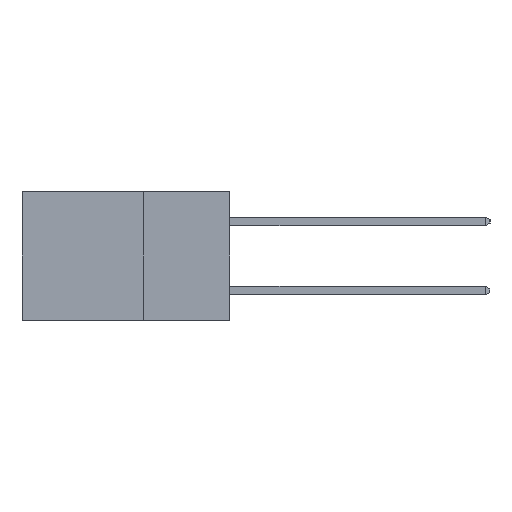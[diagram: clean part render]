
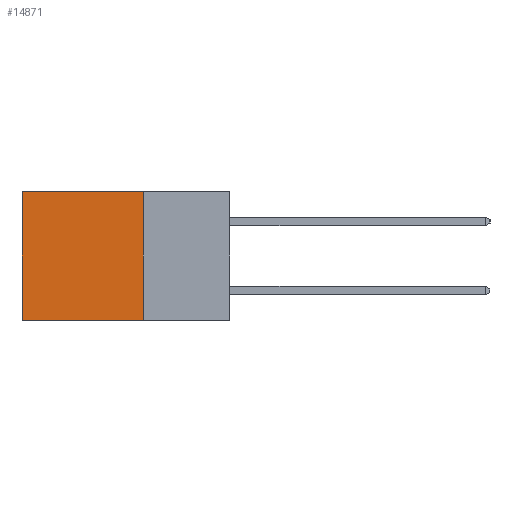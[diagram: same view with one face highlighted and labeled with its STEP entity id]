
A CAD part, left-side view. The second image highlights one B-rep face of the part: STEP entity #14871.
In plain terms, the highlighted planar face has unit normal (-1, 0, 0).
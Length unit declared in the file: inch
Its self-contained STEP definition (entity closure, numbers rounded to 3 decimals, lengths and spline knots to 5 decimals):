
#87 = LINE ( 'NONE', #19445, #12273 ) ;
#1299 = EDGE_CURVE ( 'NONE', #27703, #28392, #21581, .T. ) ;
#1652 = LINE ( 'NONE', #26095, #13767 ) ;
#2207 = CARTESIAN_POINT ( 'NONE',  ( 0.298, 0.25, 0. ) ) ;
#3709 = AXIS2_PLACEMENT_3D ( 'NONE', #2207, #4673, #21496 ) ;
#3827 = VERTEX_POINT ( 'NONE', #10806 ) ;
#4673 = DIRECTION ( 'NONE',  ( 1., 0., 0. ) ) ;
#5021 = ORIENTED_EDGE ( 'NONE', *, *, #17584, .F. ) ;
#7490 = VECTOR ( 'NONE', #25707, 39.37008 ) ;
#8195 = ORIENTED_EDGE ( 'NONE', *, *, #12023, .F. ) ;
#9973 = ORIENTED_EDGE ( 'NONE', *, *, #23979, .T. ) ;
#10806 = CARTESIAN_POINT ( 'NONE',  ( 0.298, 0.25, -0.37 ) ) ;
#12023 = EDGE_CURVE ( 'NONE', #20216, #3827, #87, .T. ) ;
#12273 = VECTOR ( 'NONE', #21855, 39.37008 ) ;
#13767 = VECTOR ( 'NONE', #28373, 39.37008 ) ;
#14640 = ORIENTED_EDGE ( 'NONE', *, *, #1299, .T. ) ;
#14871 = ADVANCED_FACE ( 'NONE', ( #19170 ), #16651, .F. ) ;
#15956 = CARTESIAN_POINT ( 'NONE',  ( 0.298, 0.25, 0. ) ) ;
#16204 = CARTESIAN_POINT ( 'NONE',  ( 0.298, 0.6, -0.37 ) ) ;
#16651 = PLANE ( 'NONE',  #3709 ) ;
#17584 = EDGE_CURVE ( 'NONE', #3827, #28392, #20247, .T. ) ;
#19170 = FACE_OUTER_BOUND ( 'NONE', #30042, .T. ) ;
#19445 = CARTESIAN_POINT ( 'NONE',  ( 0.298, 0.25, 0. ) ) ;
#20216 = VERTEX_POINT ( 'NONE', #15956 ) ;
#20247 = LINE ( 'NONE', #30378, #7490 ) ;
#21496 = DIRECTION ( 'NONE',  ( 0., 0., -1. ) ) ;
#21581 = LINE ( 'NONE', #30171, #26419 ) ;
#21855 = DIRECTION ( 'NONE',  ( 0., 0., -1. ) ) ;
#23979 = EDGE_CURVE ( 'NONE', #20216, #27703, #1652, .T. ) ;
#25707 = DIRECTION ( 'NONE',  ( 0., 1., 0. ) ) ;
#25759 = CARTESIAN_POINT ( 'NONE',  ( 0.298, 0.6, 0. ) ) ;
#26095 = CARTESIAN_POINT ( 'NONE',  ( 0.298, 0.25, 0. ) ) ;
#26419 = VECTOR ( 'NONE', #29287, 39.37008 ) ;
#27703 = VERTEX_POINT ( 'NONE', #25759 ) ;
#28373 = DIRECTION ( 'NONE',  ( 0., 1., 0. ) ) ;
#28392 = VERTEX_POINT ( 'NONE', #16204 ) ;
#29287 = DIRECTION ( 'NONE',  ( 0., 0., -1. ) ) ;
#30042 = EDGE_LOOP ( 'NONE', ( #14640, #5021, #8195, #9973 ) ) ;
#30171 = CARTESIAN_POINT ( 'NONE',  ( 0.298, 0.6, 0. ) ) ;
#30378 = CARTESIAN_POINT ( 'NONE',  ( 0.298, 0.25, -0.37 ) ) ;
